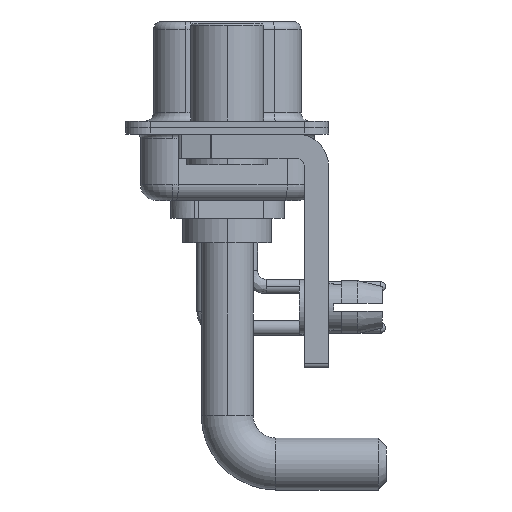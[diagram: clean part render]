
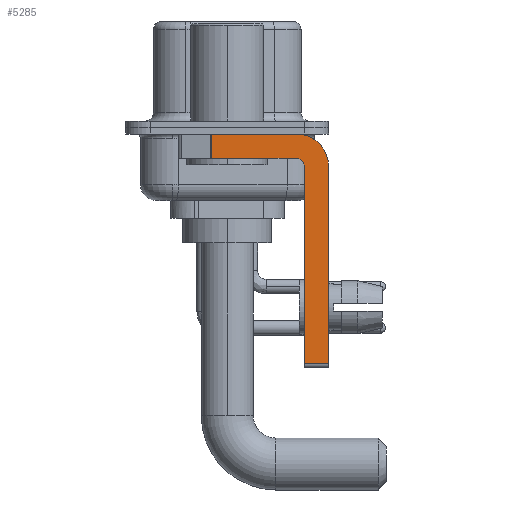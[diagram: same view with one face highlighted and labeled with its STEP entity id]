
A CAD part, left-side view. The second image highlights one B-rep face of the part: STEP entity #5285.
In plain terms, the highlighted planar face has unit normal (-1, 0, 0).
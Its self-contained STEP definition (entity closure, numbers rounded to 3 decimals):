
#186 = VECTOR ( 'NONE', #1475, 1000. ) ;
#338 = LINE ( 'NONE', #10233, #13490 ) ;
#617 = ORIENTED_EDGE ( 'NONE', *, *, #30511, .F. ) ;
#654 = DIRECTION ( 'NONE',  ( 0., 0., 1. ) ) ;
#816 = EDGE_CURVE ( 'NONE', #24119, #13746, #7117, .T. ) ;
#1130 = LINE ( 'NONE', #8461, #26292 ) ;
#1187 = EDGE_CURVE ( 'NONE', #16468, #9155, #338, .T. ) ;
#1475 = DIRECTION ( 'NONE',  ( 0., 1., 0. ) ) ;
#1625 = CARTESIAN_POINT ( 'NONE',  ( -2.9, -4.25, -1.9 ) ) ;
#2522 = VERTEX_POINT ( 'NONE', #3579 ) ;
#2912 = VERTEX_POINT ( 'NONE', #10684 ) ;
#3547 = VERTEX_POINT ( 'NONE', #20257 ) ;
#3579 = CARTESIAN_POINT ( 'NONE',  ( -2.9, -6.25, -14.55 ) ) ;
#4072 = LINE ( 'NONE', #1625, #186 ) ;
#4347 = EDGE_LOOP ( 'NONE', ( #15636, #10288, #617, #9691, #11522, #28021, #21230, #7295 ) ) ;
#4351 = CARTESIAN_POINT ( 'NONE',  ( -2.9, -4.25, -2.4 ) ) ;
#5285 = ADVANCED_FACE ( 'NONE', ( #11646 ), #26552, .F. ) ;
#5752 = DIRECTION ( 'NONE',  ( 0., 0., -1. ) ) ;
#7117 = CIRCLE ( 'NONE', #26780, 2. ) ;
#7262 = EDGE_CURVE ( 'NONE', #16468, #24119, #11344, .T. ) ;
#7295 = ORIENTED_EDGE ( 'NONE', *, *, #816, .F. ) ;
#8461 = CARTESIAN_POINT ( 'NONE',  ( -2.9, -4.75, -14.8 ) ) ;
#8483 = VECTOR ( 'NONE', #5752, 1000. ) ;
#8519 = LINE ( 'NONE', #23577, #8483 ) ;
#8650 = DIRECTION ( 'NONE',  ( 0., 0., -1. ) ) ;
#8796 = DIRECTION ( 'NONE',  ( 1., 0., 0. ) ) ;
#8940 = VECTOR ( 'NONE', #28708, 1000. ) ;
#9155 = VERTEX_POINT ( 'NONE', #12410 ) ;
#9691 = ORIENTED_EDGE ( 'NONE', *, *, #15652, .F. ) ;
#10233 = CARTESIAN_POINT ( 'NONE',  ( -2.9, 0.978, -1.9 ) ) ;
#10288 = ORIENTED_EDGE ( 'NONE', *, *, #1187, .T. ) ;
#10652 = DIRECTION ( 'NONE',  ( 0., 0., 1. ) ) ;
#10684 = CARTESIAN_POINT ( 'NONE',  ( -2.9, -4.25, -1.9 ) ) ;
#11344 = LINE ( 'NONE', #19270, #29477 ) ;
#11522 = ORIENTED_EDGE ( 'NONE', *, *, #21127, .F. ) ;
#11646 = FACE_OUTER_BOUND ( 'NONE', #4347, .T. ) ;
#11860 = EDGE_CURVE ( 'NONE', #3547, #2522, #23689, .T. ) ;
#12410 = CARTESIAN_POINT ( 'NONE',  ( -2.9, 0.978, -1.9 ) ) ;
#13365 = VERTEX_POINT ( 'NONE', #18795 ) ;
#13490 = VECTOR ( 'NONE', #27575, 1000. ) ;
#13746 = VERTEX_POINT ( 'NONE', #23007 ) ;
#13871 = CARTESIAN_POINT ( 'NONE',  ( -2.9, -4.25, -2.4 ) ) ;
#14840 = CARTESIAN_POINT ( 'NONE',  ( -2.9, 0.978, -0.4 ) ) ;
#15636 = ORIENTED_EDGE ( 'NONE', *, *, #7262, .F. ) ;
#15652 = EDGE_CURVE ( 'NONE', #13365, #2912, #30692, .T. ) ;
#15952 = EDGE_CURVE ( 'NONE', #13746, #2522, #8519, .T. ) ;
#16468 = VERTEX_POINT ( 'NONE', #14840 ) ;
#16667 = DIRECTION ( 'NONE',  ( 0., -1., 0. ) ) ;
#18795 = CARTESIAN_POINT ( 'NONE',  ( -2.9, -4.75, -2.4 ) ) ;
#19270 = CARTESIAN_POINT ( 'NONE',  ( -2.9, 3., -0.4 ) ) ;
#19577 = DIRECTION ( 'NONE',  ( 0., 0., -1. ) ) ;
#20107 = CARTESIAN_POINT ( 'NONE',  ( -2.9, -4.25, -0.4 ) ) ;
#20257 = CARTESIAN_POINT ( 'NONE',  ( -2.9, -4.75, -14.55 ) ) ;
#21127 = EDGE_CURVE ( 'NONE', #3547, #13365, #1130, .T. ) ;
#21230 = ORIENTED_EDGE ( 'NONE', *, *, #15952, .F. ) ;
#22944 = CARTESIAN_POINT ( 'NONE',  ( -2.9, -4.25, -2.4 ) ) ;
#23007 = CARTESIAN_POINT ( 'NONE',  ( -2.9, -6.25, -2.4 ) ) ;
#23577 = CARTESIAN_POINT ( 'NONE',  ( -2.9, -6.25, -2.4 ) ) ;
#23689 = LINE ( 'NONE', #25957, #8940 ) ;
#23758 = DIRECTION ( 'NONE',  ( -1., 0., 0. ) ) ;
#24119 = VERTEX_POINT ( 'NONE', #20107 ) ;
#24123 = DIRECTION ( 'NONE',  ( 1., 0., 0. ) ) ;
#25125 = AXIS2_PLACEMENT_3D ( 'NONE', #4351, #24123, #19577 ) ;
#25957 = CARTESIAN_POINT ( 'NONE',  ( -2.9, -4.25, -14.55 ) ) ;
#26292 = VECTOR ( 'NONE', #654, 1000. ) ;
#26552 = PLANE ( 'NONE',  #25125 ) ;
#26780 = AXIS2_PLACEMENT_3D ( 'NONE', #22944, #8796, #8650 ) ;
#27575 = DIRECTION ( 'NONE',  ( 0., 0., -1. ) ) ;
#28021 = ORIENTED_EDGE ( 'NONE', *, *, #11860, .T. ) ;
#28708 = DIRECTION ( 'NONE',  ( 0., -1., 0. ) ) ;
#29477 = VECTOR ( 'NONE', #16667, 1000. ) ;
#29685 = AXIS2_PLACEMENT_3D ( 'NONE', #13871, #23758, #10652 ) ;
#30511 = EDGE_CURVE ( 'NONE', #2912, #9155, #4072, .T. ) ;
#30692 = CIRCLE ( 'NONE', #29685, 0.5 ) ;
